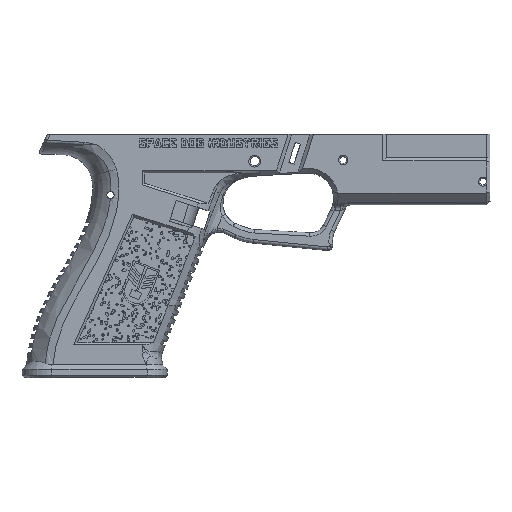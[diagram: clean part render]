
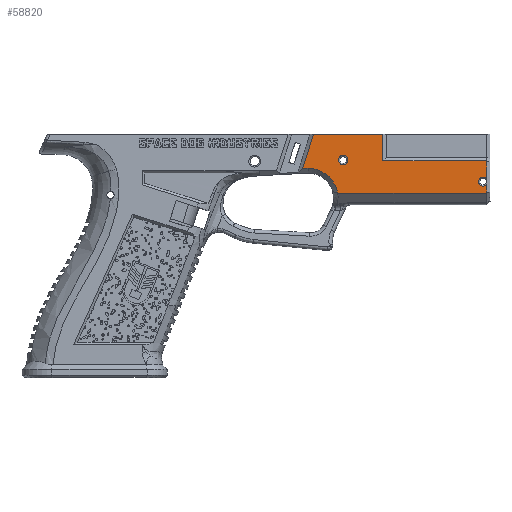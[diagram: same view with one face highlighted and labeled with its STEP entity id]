
A CAD part, top view. The second image highlights one B-rep face of the part: STEP entity #58820.
In plain terms, the highlighted planar face has unit normal (0, 0, 1).
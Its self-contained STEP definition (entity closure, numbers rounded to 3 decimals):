
#423=FACE_BOUND('',#15716,.T.);
#8712=PLANE('',#60245);
#11912=FACE_OUTER_BOUND('',#15715,.T.);
#15715=EDGE_LOOP('',(#52531,#52532,#52533,#52534,#52535,#52536,#52537,#52538,
#52539,#52540,#52541));
#15716=EDGE_LOOP('',(#52542));
#18677=LINE('',#118069,#22228);
#18679=LINE('',#118076,#22230);
#18680=LINE('',#118094,#22231);
#18681=LINE('',#118095,#22232);
#19219=LINE('',#128863,#22770);
#19220=LINE('',#128866,#22771);
#19221=LINE('',#128868,#22772);
#19222=LINE('',#128869,#22773);
#22228=VECTOR('',#64692,10.);
#22230=VECTOR('',#64696,10.);
#22231=VECTOR('',#64699,10.);
#22232=VECTOR('',#64700,10.);
#22770=VECTOR('',#65604,10.);
#22771=VECTOR('',#65607,10.);
#22772=VECTOR('',#65608,10.);
#22773=VECTOR('',#65609,10.);
#23369=CIRCLE('',#60064,2.);
#23370=CIRCLE('',#60065,2.);
#23372=CIRCLE('',#60068,2.025);
#23382=CIRCLE('',#60113,13.);
#25774=VERTEX_POINT('',#86735);
#25776=VERTEX_POINT('',#86741);
#27885=VERTEX_POINT('',#118068);
#27886=VERTEX_POINT('',#118074);
#27887=VERTEX_POINT('',#118078);
#27888=VERTEX_POINT('',#118079);
#27889=VERTEX_POINT('',#118097);
#27890=VERTEX_POINT('',#118102);
#28560=VERTEX_POINT('',#124169);
#28723=VERTEX_POINT('',#128861);
#28724=VERTEX_POINT('',#128865);
#28725=VERTEX_POINT('',#128867);
#35890=EDGE_CURVE('',#25776,#27885,#18677,.T.);
#35893=EDGE_CURVE('',#25774,#27886,#18679,.T.);
#35895=EDGE_CURVE('',#27887,#25776,#18680,.T.);
#35896=EDGE_CURVE('',#25774,#27888,#18681,.T.);
#35898=EDGE_CURVE('',#27889,#27887,#23369,.T.);
#35899=EDGE_CURVE('',#27888,#27889,#23370,.T.);
#35901=EDGE_CURVE('',#27890,#27890,#23372,.T.);
#36808=EDGE_CURVE('',#27885,#28560,#23382,.T.);
#37148=EDGE_CURVE('',#28723,#27886,#19219,.T.);
#37149=EDGE_CURVE('',#28724,#28723,#19220,.T.);
#37150=EDGE_CURVE('',#28725,#28724,#19221,.T.);
#37151=EDGE_CURVE('',#28560,#28725,#19222,.T.);
#52531=ORIENTED_EDGE('',*,*,#35899,.F.);
#52532=ORIENTED_EDGE('',*,*,#35896,.F.);
#52533=ORIENTED_EDGE('',*,*,#35893,.T.);
#52534=ORIENTED_EDGE('',*,*,#37148,.F.);
#52535=ORIENTED_EDGE('',*,*,#37149,.F.);
#52536=ORIENTED_EDGE('',*,*,#37150,.F.);
#52537=ORIENTED_EDGE('',*,*,#37151,.F.);
#52538=ORIENTED_EDGE('',*,*,#36808,.F.);
#52539=ORIENTED_EDGE('',*,*,#35890,.F.);
#52540=ORIENTED_EDGE('',*,*,#35895,.F.);
#52541=ORIENTED_EDGE('',*,*,#35898,.F.);
#52542=ORIENTED_EDGE('',*,*,#35901,.T.);
#58820=ADVANCED_FACE('',(#11912,#423),#8712,.F.);
#60064=AXIS2_PLACEMENT_3D('',#118099,#64705,#64706);
#60065=AXIS2_PLACEMENT_3D('',#118100,#64707,#64708);
#60068=AXIS2_PLACEMENT_3D('',#118104,#64713,#64714);
#60113=AXIS2_PLACEMENT_3D('',#124170,#65118,#65119);
#60245=AXIS2_PLACEMENT_3D('',#128864,#65605,#65606);
#64692=DIRECTION('',(-1.,0.,0.));
#64696=DIRECTION('',(-1.,0.,0.));
#64699=DIRECTION('',(0.,-1.,0.));
#64700=DIRECTION('',(0.,-1.,0.));
#64705=DIRECTION('center_axis',(0.,0.,
1.));
#64706=DIRECTION('ref_axis',(-1.,0.,0.));
#64707=DIRECTION('center_axis',(0.,0.,
1.));
#64708=DIRECTION('ref_axis',(-1.,0.,0.));
#64713=DIRECTION('center_axis',(0.,0.,
-1.));
#64714=DIRECTION('ref_axis',(0.776,-0.63,0.));
#65118=DIRECTION('center_axis',(0.,0.,
1.));
#65119=DIRECTION('ref_axis',(0.892,-0.452,0.));
#65604=DIRECTION('',(0.,-1.,0.));
#65605=DIRECTION('center_axis',(0.,0.,
-1.));
#65606=DIRECTION('ref_axis',(0.,1.,0.));
#65607=DIRECTION('',(1.,0.,0.));
#65608=DIRECTION('',(0.301,0.954,0.));
#65609=DIRECTION('',(-0.999,-0.055,0.));
#86735=CARTESIAN_POINT('',(157.635,-9.733,23.145));
#86741=CARTESIAN_POINT('',(157.635,-23.787,23.145));
#118068=CARTESIAN_POINT('',(93.078,-23.787,23.145));
#118069=CARTESIAN_POINT('',(89.618,-23.787,23.145));
#118074=CARTESIAN_POINT('',(112.635,-9.733,23.145));
#118076=CARTESIAN_POINT('',(105.549,-9.733,23.145));
#118078=CARTESIAN_POINT('',(157.635,-20.11,23.145));
#118079=CARTESIAN_POINT('',(157.635,-17.464,23.145));
#118094=CARTESIAN_POINT('',(157.635,-25.087,23.145));
#118095=CARTESIAN_POINT('',(157.635,-25.087,23.145));
#118097=CARTESIAN_POINT('',(154.135,-18.787,23.145));
#118099=CARTESIAN_POINT('Origin',(156.135,-18.787,23.145));
#118100=CARTESIAN_POINT('Origin',(156.135,-18.787,23.145));
#118102=CARTESIAN_POINT('',(97.469,-9.398,23.145));
#118104=CARTESIAN_POINT('Origin',(95.444,-9.398,23.145));
#124169=CARTESIAN_POINT('',(80.217,-13.037,23.145));
#124170=CARTESIAN_POINT('Origin',(80.274,-26.037,23.145));
#128861=CARTESIAN_POINT('',(112.635,1.767,23.145));
#128863=CARTESIAN_POINT('',(112.635,1.513,23.145));
#128864=CARTESIAN_POINT('Origin',(103.31,1.259,23.145));
#128865=CARTESIAN_POINT('',(82.591,1.767,23.145));
#128866=CARTESIAN_POINT('',(33.317,1.767,23.145));
#128867=CARTESIAN_POINT('',(77.883,-13.165,23.145));
#128868=CARTESIAN_POINT('',(82.185,0.48,23.145));
#128869=CARTESIAN_POINT('',(81.633,-12.959,23.145));
